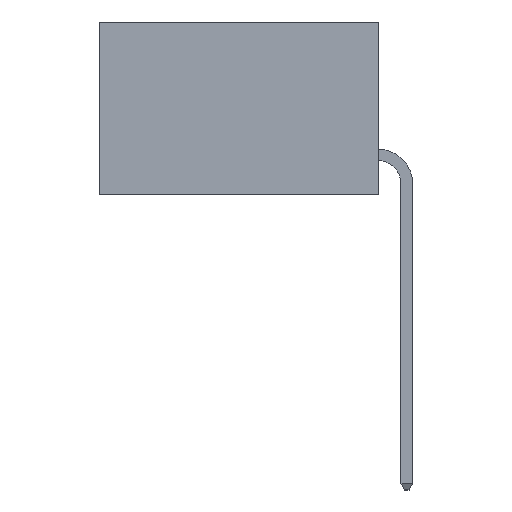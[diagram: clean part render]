
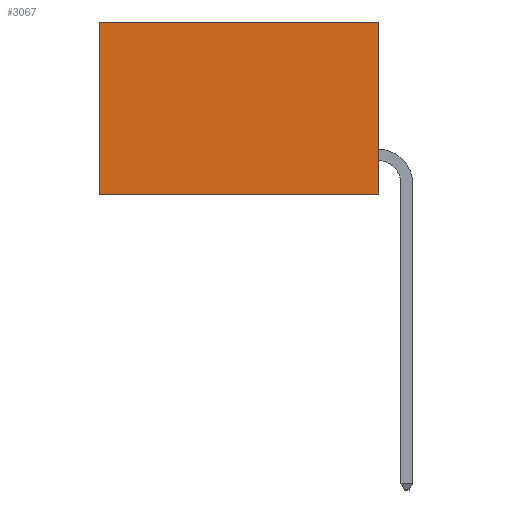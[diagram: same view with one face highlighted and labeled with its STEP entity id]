
A CAD part, left-side view. The second image highlights one B-rep face of the part: STEP entity #3067.
In plain terms, the highlighted planar face has unit normal (-1, 0, 0).
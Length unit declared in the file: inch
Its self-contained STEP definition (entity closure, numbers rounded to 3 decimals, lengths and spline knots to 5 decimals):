
#555 = VERTEX_POINT ( 'NONE', #5198 ) ;
#713 = LINE ( 'NONE', #8797, #4921 ) ;
#803 = CARTESIAN_POINT ( 'NONE',  ( 0.2615, 0., 0. ) ) ;
#829 = DIRECTION ( 'NONE',  ( 0., 1., 0. ) ) ;
#1216 = EDGE_CURVE ( 'NONE', #3380, #555, #10433, .T. ) ;
#1394 = EDGE_CURVE ( 'NONE', #3380, #9348, #3913, .T. ) ;
#1983 = DIRECTION ( 'NONE',  ( 0., 0., -1. ) ) ;
#2062 = DIRECTION ( 'NONE',  ( 1., 0., 0. ) ) ;
#2196 = CARTESIAN_POINT ( 'NONE',  ( 0.2615, 0., -0.37 ) ) ;
#2753 = PLANE ( 'NONE',  #3683 ) ;
#2801 = VERTEX_POINT ( 'NONE', #6160 ) ;
#3067 = ADVANCED_FACE ( 'NONE', ( #9590 ), #2753, .F. ) ;
#3250 = CARTESIAN_POINT ( 'NONE',  ( 0.2615, 0., -0.37 ) ) ;
#3380 = VERTEX_POINT ( 'NONE', #8782 ) ;
#3490 = DIRECTION ( 'NONE',  ( 0., 1., 0. ) ) ;
#3683 = AXIS2_PLACEMENT_3D ( 'NONE', #2196, #2062, #1983 ) ;
#3913 = LINE ( 'NONE', #10354, #7986 ) ;
#4619 = EDGE_LOOP ( 'NONE', ( #8959, #8974, #8992, #9008 ) ) ;
#4921 = VECTOR ( 'NONE', #8225, 39.37008 ) ;
#5062 = CARTESIAN_POINT ( 'NONE',  ( 0.2615, 0., -0.37 ) ) ;
#5198 = CARTESIAN_POINT ( 'NONE',  ( 0.2615, 0.6, 0. ) ) ;
#6160 = CARTESIAN_POINT ( 'NONE',  ( 0.2615, 0.6, -0.37 ) ) ;
#6285 = LINE ( 'NONE', #3250, #10062 ) ;
#7595 = EDGE_CURVE ( 'NONE', #555, #2801, #713, .T. ) ;
#7672 = EDGE_CURVE ( 'NONE', #9348, #2801, #6285, .T. ) ;
#7986 = VECTOR ( 'NONE', #10465, 39.37008 ) ;
#8225 = DIRECTION ( 'NONE',  ( 0., 0., -1. ) ) ;
#8396 = VECTOR ( 'NONE', #829, 39.37008 ) ;
#8782 = CARTESIAN_POINT ( 'NONE',  ( 0.2615, 0., 0. ) ) ;
#8797 = CARTESIAN_POINT ( 'NONE',  ( 0.2615, 0.6, -0.37 ) ) ;
#8959 = ORIENTED_EDGE ( 'NONE', *, *, #7595, .T. ) ;
#8974 = ORIENTED_EDGE ( 'NONE', *, *, #7672, .F. ) ;
#8992 = ORIENTED_EDGE ( 'NONE', *, *, #1394, .F. ) ;
#9008 = ORIENTED_EDGE ( 'NONE', *, *, #1216, .T. ) ;
#9348 = VERTEX_POINT ( 'NONE', #5062 ) ;
#9590 = FACE_OUTER_BOUND ( 'NONE', #4619, .T. ) ;
#10062 = VECTOR ( 'NONE', #3490, 39.37008 ) ;
#10354 = CARTESIAN_POINT ( 'NONE',  ( 0.2615, 0., -0.37 ) ) ;
#10433 = LINE ( 'NONE', #803, #8396 ) ;
#10465 = DIRECTION ( 'NONE',  ( 0., 0., -1. ) ) ;
